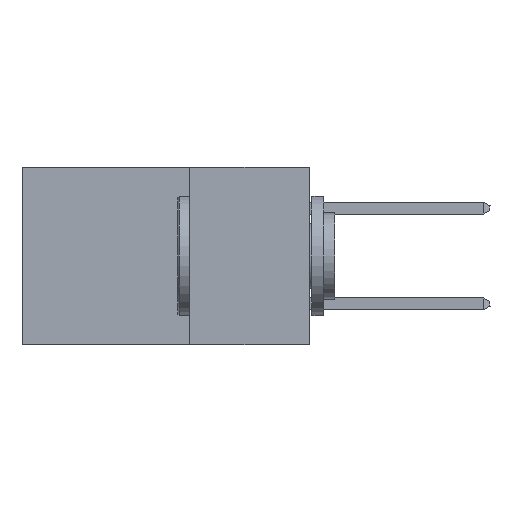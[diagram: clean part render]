
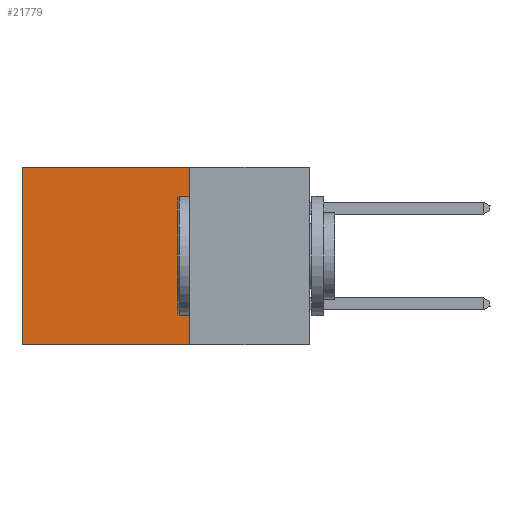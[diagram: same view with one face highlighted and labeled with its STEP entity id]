
A CAD part, left-side view. The second image highlights one B-rep face of the part: STEP entity #21779.
In plain terms, the highlighted planar face has unit normal (-1, 0, 0).
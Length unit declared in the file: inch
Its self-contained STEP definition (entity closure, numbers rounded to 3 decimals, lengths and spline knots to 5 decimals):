
#62 = LINE ( 'NONE', #25092, #10271 ) ;
#552 = ORIENTED_EDGE ( 'NONE', *, *, #22789, .T. ) ;
#1280 = ORIENTED_EDGE ( 'NONE', *, *, #3817, .T. ) ;
#1532 = VERTEX_POINT ( 'NONE', #32972 ) ;
#1595 = CARTESIAN_POINT ( 'NONE',  ( 0.2875, 0.25, 0. ) ) ;
#2062 = AXIS2_PLACEMENT_3D ( 'NONE', #34638, #18053, #11920 ) ;
#2371 = VECTOR ( 'NONE', #15188, 39.37008 ) ;
#3815 = CARTESIAN_POINT ( 'NONE',  ( 0.2875, 0.25, -0.37 ) ) ;
#3817 = EDGE_CURVE ( 'NONE', #26850, #31579, #10476, .T. ) ;
#4241 = VERTEX_POINT ( 'NONE', #23196 ) ;
#4850 = DIRECTION ( 'NONE',  ( 0., 1., 0. ) ) ;
#5630 = LINE ( 'NONE', #1595, #13637 ) ;
#6133 = EDGE_CURVE ( 'NONE', #1532, #31579, #34856, .T. ) ;
#7245 = ORIENTED_EDGE ( 'NONE', *, *, #6133, .F. ) ;
#7297 = ORIENTED_EDGE ( 'NONE', *, *, #24724, .F. ) ;
#10271 = VECTOR ( 'NONE', #16826, 39.37008 ) ;
#10476 = LINE ( 'NONE', #11353, #13141 ) ;
#11353 = CARTESIAN_POINT ( 'NONE',  ( 0.2875, 0.6, 0. ) ) ;
#11920 = DIRECTION ( 'NONE',  ( 0., 0., -1. ) ) ;
#13141 = VECTOR ( 'NONE', #23782, 39.37008 ) ;
#13637 = VECTOR ( 'NONE', #4850, 39.37008 ) ;
#15188 = DIRECTION ( 'NONE',  ( 0., 1., 0. ) ) ;
#16826 = DIRECTION ( 'NONE',  ( 0., 0., -1. ) ) ;
#18053 = DIRECTION ( 'NONE',  ( 1., 0., 0. ) ) ;
#18946 = EDGE_LOOP ( 'NONE', ( #1280, #7245, #7297, #552 ) ) ;
#19444 = CARTESIAN_POINT ( 'NONE',  ( 0.2875, 0.6, 0. ) ) ;
#21355 = CARTESIAN_POINT ( 'NONE',  ( 0.2875, 0.6, -0.37 ) ) ;
#21779 = ADVANCED_FACE ( 'NONE', ( #23931 ), #32060, .F. ) ;
#22789 = EDGE_CURVE ( 'NONE', #4241, #26850, #5630, .T. ) ;
#23196 = CARTESIAN_POINT ( 'NONE',  ( 0.2875, 0.25, 0. ) ) ;
#23782 = DIRECTION ( 'NONE',  ( 0., 0., -1. ) ) ;
#23931 = FACE_OUTER_BOUND ( 'NONE', #18946, .T. ) ;
#24724 = EDGE_CURVE ( 'NONE', #4241, #1532, #62, .T. ) ;
#25092 = CARTESIAN_POINT ( 'NONE',  ( 0.2875, 0.25, 0. ) ) ;
#26850 = VERTEX_POINT ( 'NONE', #19444 ) ;
#31579 = VERTEX_POINT ( 'NONE', #21355 ) ;
#32060 = PLANE ( 'NONE',  #2062 ) ;
#32972 = CARTESIAN_POINT ( 'NONE',  ( 0.2875, 0.25, -0.37 ) ) ;
#34638 = CARTESIAN_POINT ( 'NONE',  ( 0.2875, 0.25, 0. ) ) ;
#34856 = LINE ( 'NONE', #3815, #2371 ) ;
